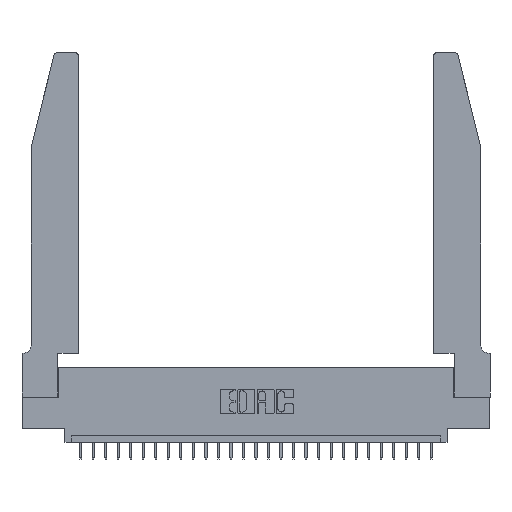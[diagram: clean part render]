
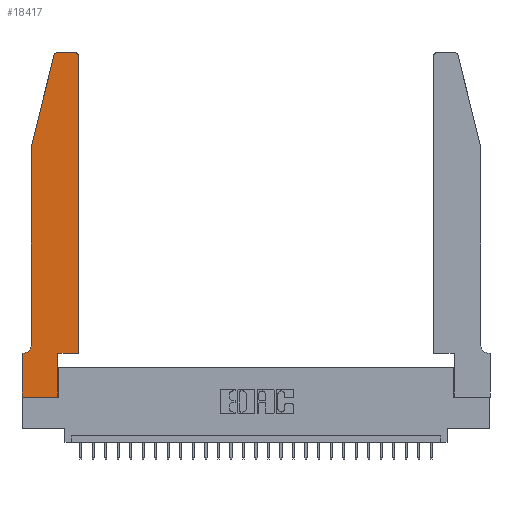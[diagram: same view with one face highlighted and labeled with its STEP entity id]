
A CAD part, top view. The second image highlights one B-rep face of the part: STEP entity #18417.
In plain terms, the highlighted planar face has unit normal (0, 0, 1).
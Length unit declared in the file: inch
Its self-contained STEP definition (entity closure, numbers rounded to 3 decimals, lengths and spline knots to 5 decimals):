
#150 = ORIENTED_EDGE ( 'NONE', *, *, #7265, .T. ) ;
#175 = DIRECTION ( 'NONE',  ( 0., -1., 0. ) ) ;
#568 = VECTOR ( 'NONE', #13580, 39.37008 ) ;
#1531 = EDGE_CURVE ( 'NONE', #26109, #5052, #18357, .T. ) ;
#1539 = VERTEX_POINT ( 'NONE', #25055 ) ;
#1590 = DIRECTION ( 'NONE',  ( 0., 1., 0. ) ) ;
#2040 = EDGE_CURVE ( 'NONE', #5052, #1539, #27273, .T. ) ;
#2103 = ORIENTED_EDGE ( 'NONE', *, *, #14664, .T. ) ;
#2546 = PLANE ( 'NONE',  #24743 ) ;
#2674 = DIRECTION ( 'NONE',  ( 1., 0., 0. ) ) ;
#3276 = DIRECTION ( 'NONE',  ( -1., 0., 0. ) ) ;
#3424 = LINE ( 'NONE', #12406, #12288 ) ;
#3772 = LINE ( 'NONE', #25290, #13368 ) ;
#4177 = CARTESIAN_POINT ( 'NONE',  ( 0.0755, 2., 0.37 ) ) ;
#4531 = LINE ( 'NONE', #13358, #21961 ) ;
#4620 = VECTOR ( 'NONE', #8588, 39.37008 ) ;
#5052 = VERTEX_POINT ( 'NONE', #12667 ) ;
#5104 = ORIENTED_EDGE ( 'NONE', *, *, #21609, .T. ) ;
#5205 = EDGE_CURVE ( 'NONE', #5380, #25213, #21727, .T. ) ;
#5380 = VERTEX_POINT ( 'NONE', #23136 ) ;
#5768 = EDGE_CURVE ( 'NONE', #12040, #15312, #12510, .T. ) ;
#6491 = FACE_OUTER_BOUND ( 'NONE', #27118, .T. ) ;
#6578 = CARTESIAN_POINT ( 'NONE',  ( 0.0755, 2., 0.37 ) ) ;
#7265 = EDGE_CURVE ( 'NONE', #16162, #19671, #4531, .T. ) ;
#7436 = LINE ( 'NONE', #20422, #12233 ) ;
#7499 = CARTESIAN_POINT ( 'NONE',  ( 0.2605, 2.75, 0.37 ) ) ;
#7613 = DIRECTION ( 'NONE',  ( 0., 0., -1. ) ) ;
#7617 = CARTESIAN_POINT ( 'NONE',  ( 0., 0., 0.37 ) ) ;
#7748 = AXIS2_PLACEMENT_3D ( 'NONE', #8634, #22441, #2674 ) ;
#8130 = ORIENTED_EDGE ( 'NONE', *, *, #5205, .T. ) ;
#8588 = DIRECTION ( 'NONE',  ( 0., 1., 0. ) ) ;
#8634 = CARTESIAN_POINT ( 'NONE',  ( 0.4205, 2.72, 0.37 ) ) ;
#9239 = DIRECTION ( 'NONE',  ( -1., 0., 0. ) ) ;
#9540 = AXIS2_PLACEMENT_3D ( 'NONE', #18595, #7613, #3276 ) ;
#9673 = CARTESIAN_POINT ( 'NONE',  ( 0.0755, 0.35, 0.37 ) ) ;
#9895 = EDGE_CURVE ( 'NONE', #25213, #22951, #3424, .T. ) ;
#10134 = VECTOR ( 'NONE', #15121, 39.37008 ) ;
#11584 = ORIENTED_EDGE ( 'NONE', *, *, #5768, .T. ) ;
#12040 = VERTEX_POINT ( 'NONE', #24240 ) ;
#12140 = EDGE_CURVE ( 'NONE', #23623, #16162, #20059, .T. ) ;
#12156 = ORIENTED_EDGE ( 'NONE', *, *, #9895, .T. ) ;
#12233 = VECTOR ( 'NONE', #22417, 39.37008 ) ;
#12288 = VECTOR ( 'NONE', #14554, 39.37008 ) ;
#12406 = CARTESIAN_POINT ( 'NONE',  ( 0.0755, 2., 0.37 ) ) ;
#12510 = LINE ( 'NONE', #12794, #4620 ) ;
#12637 = EDGE_CURVE ( 'NONE', #1539, #5380, #24576, .T. ) ;
#12667 = CARTESIAN_POINT ( 'NONE',  ( 0.4205, 2.75, 0.37 ) ) ;
#12794 = CARTESIAN_POINT ( 'NONE',  ( 0.2865, 0.35, 0.37 ) ) ;
#13358 = CARTESIAN_POINT ( 'NONE',  ( 0., 0., 0.37 ) ) ;
#13368 = VECTOR ( 'NONE', #1590, 39.37008 ) ;
#13580 = DIRECTION ( 'NONE',  ( -1., 0., 0. ) ) ;
#13688 = DIRECTION ( 'NONE',  ( 0., 0., 1. ) ) ;
#13917 = CARTESIAN_POINT ( 'NONE',  ( 0., 0.35, 0.37 ) ) ;
#14242 = VECTOR ( 'NONE', #9239, 39.37008 ) ;
#14554 = DIRECTION ( 'NONE',  ( 0., -1., 0. ) ) ;
#14664 = EDGE_CURVE ( 'NONE', #19671, #12040, #7436, .T. ) ;
#15121 = DIRECTION ( 'NONE',  ( -0.239, -0.971, 0. ) ) ;
#15312 = VERTEX_POINT ( 'NONE', #18188 ) ;
#15426 = DIRECTION ( 'NONE',  ( 0., 0., 1. ) ) ;
#15863 = DIRECTION ( 'NONE',  ( 1., 0., 0. ) ) ;
#16162 = VERTEX_POINT ( 'NONE', #13917 ) ;
#16273 = VERTEX_POINT ( 'NONE', #18654 ) ;
#16300 = ORIENTED_EDGE ( 'NONE', *, *, #12140, .T. ) ;
#16587 = EDGE_CURVE ( 'NONE', #15312, #16273, #23210, .T. ) ;
#17392 = VECTOR ( 'NONE', #19197, 39.37008 ) ;
#17868 = DIRECTION ( 'NONE',  ( 1., 0., 0. ) ) ;
#18188 = CARTESIAN_POINT ( 'NONE',  ( 0.2865, 0.35, 0.37 ) ) ;
#18357 = CIRCLE ( 'NONE', #7748, 0.03 ) ;
#18417 = ADVANCED_FACE ( 'NONE', ( #6491 ), #2546, .T. ) ;
#18526 = EDGE_CURVE ( 'NONE', #22951, #23623, #27049, .T. ) ;
#18595 = CARTESIAN_POINT ( 'NONE',  ( 0.0055, 0.42, 0.37 ) ) ;
#18654 = CARTESIAN_POINT ( 'NONE',  ( 0.4505, 0.35, 0.37 ) ) ;
#19197 = DIRECTION ( 'NONE',  ( 1., 0., 0. ) ) ;
#19268 = CARTESIAN_POINT ( 'NONE',  ( 0.0755, 0.42, 0.37 ) ) ;
#19671 = VERTEX_POINT ( 'NONE', #7617 ) ;
#19735 = ORIENTED_EDGE ( 'NONE', *, *, #2040, .T. ) ;
#19875 = CARTESIAN_POINT ( 'NONE',  ( 0.4505, 2.72, 0.37 ) ) ;
#20059 = LINE ( 'NONE', #9673, #568 ) ;
#20422 = CARTESIAN_POINT ( 'NONE',  ( 0., 0., 0.37 ) ) ;
#21254 = ORIENTED_EDGE ( 'NONE', *, *, #12637, .T. ) ;
#21609 = EDGE_CURVE ( 'NONE', #16273, #26109, #3772, .T. ) ;
#21727 = LINE ( 'NONE', #6578, #10134 ) ;
#21961 = VECTOR ( 'NONE', #175, 39.37008 ) ;
#22412 = ORIENTED_EDGE ( 'NONE', *, *, #1531, .T. ) ;
#22417 = DIRECTION ( 'NONE',  ( 1., 0., 0. ) ) ;
#22441 = DIRECTION ( 'NONE',  ( 0., 0., 1. ) ) ;
#22951 = VERTEX_POINT ( 'NONE', #19268 ) ;
#23136 = CARTESIAN_POINT ( 'NONE',  ( 0.25487, 2.72718, 0.37 ) ) ;
#23210 = LINE ( 'NONE', #23515, #17392 ) ;
#23338 = ORIENTED_EDGE ( 'NONE', *, *, #18526, .T. ) ;
#23515 = CARTESIAN_POINT ( 'NONE',  ( 0.4505, 0.35, 0.37 ) ) ;
#23623 = VERTEX_POINT ( 'NONE', #27378 ) ;
#24240 = CARTESIAN_POINT ( 'NONE',  ( 0.2865, 0., 0.37 ) ) ;
#24358 = CARTESIAN_POINT ( 'NONE',  ( 0.284, 2.72, 0.37 ) ) ;
#24576 = CIRCLE ( 'NONE', #25037, 0.03 ) ;
#24743 = AXIS2_PLACEMENT_3D ( 'NONE', #26397, #15426, #15863 ) ;
#25037 = AXIS2_PLACEMENT_3D ( 'NONE', #24358, #13688, #17868 ) ;
#25055 = CARTESIAN_POINT ( 'NONE',  ( 0.284, 2.75, 0.37 ) ) ;
#25213 = VERTEX_POINT ( 'NONE', #4177 ) ;
#25290 = CARTESIAN_POINT ( 'NONE',  ( 0.4505, 0.35, 0.37 ) ) ;
#26109 = VERTEX_POINT ( 'NONE', #19875 ) ;
#26397 = CARTESIAN_POINT ( 'NONE',  ( 0., 0.35, 0.37 ) ) ;
#27049 = CIRCLE ( 'NONE', #9540, 0.07 ) ;
#27118 = EDGE_LOOP ( 'NONE', ( #19735, #21254, #8130, #12156, #23338, #16300, #150, #2103, #11584, #27233, #5104, #22412 ) ) ;
#27233 = ORIENTED_EDGE ( 'NONE', *, *, #16587, .T. ) ;
#27273 = LINE ( 'NONE', #7499, #14242 ) ;
#27378 = CARTESIAN_POINT ( 'NONE',  ( 0.0055, 0.35, 0.37 ) ) ;
